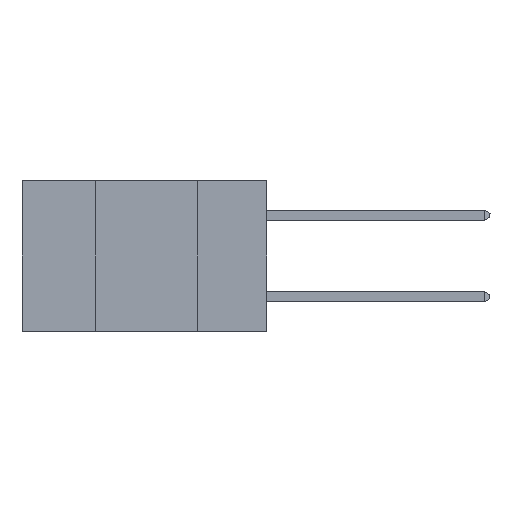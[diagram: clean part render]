
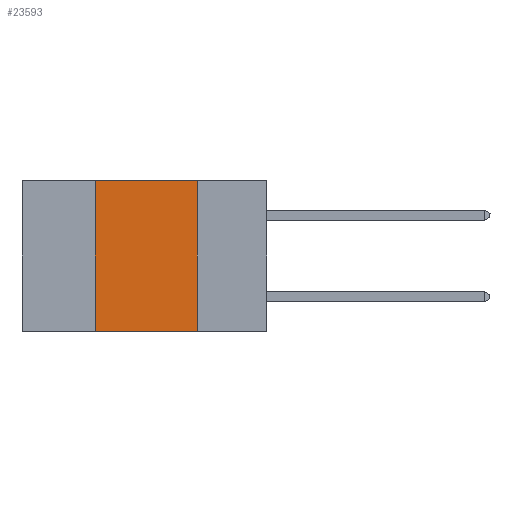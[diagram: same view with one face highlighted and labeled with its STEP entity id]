
A CAD part, left-side view. The second image highlights one B-rep face of the part: STEP entity #23593.
In plain terms, the highlighted planar face has unit normal (-1, 0, 0).
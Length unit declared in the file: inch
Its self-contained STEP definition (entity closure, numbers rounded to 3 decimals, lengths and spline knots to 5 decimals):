
#224 = EDGE_CURVE ( 'NONE', #19193, #25622, #569, .T. ) ;
#418 = ORIENTED_EDGE ( 'NONE', *, *, #20161, .F. ) ;
#569 = LINE ( 'NONE', #13970, #28613 ) ;
#1901 = CARTESIAN_POINT ( 'NONE',  ( 0., 0.42, -0.37 ) ) ;
#2568 = CARTESIAN_POINT ( 'NONE',  ( 0., 0.17, -0.37 ) ) ;
#2812 = EDGE_LOOP ( 'NONE', ( #418, #16305, #35563, #21832 ) ) ;
#4475 = CARTESIAN_POINT ( 'NONE',  ( 0., 0.6, 0. ) ) ;
#4681 = EDGE_CURVE ( 'NONE', #19193, #18682, #34011, .T. ) ;
#4736 = DIRECTION ( 'NONE',  ( 0., 0., -1. ) ) ;
#6014 = DIRECTION ( 'NONE',  ( 0., 0., -1. ) ) ;
#7960 = CARTESIAN_POINT ( 'NONE',  ( 0., 0.42, 0. ) ) ;
#8707 = CARTESIAN_POINT ( 'NONE',  ( 0., 0.17, 0. ) ) ;
#9124 = CARTESIAN_POINT ( 'NONE',  ( 0., 0.6, -0.37 ) ) ;
#9459 = CARTESIAN_POINT ( 'NONE',  ( 0., 0.17, 0. ) ) ;
#9792 = EDGE_CURVE ( 'NONE', #25622, #32981, #25194, .T. ) ;
#10490 = DIRECTION ( 'NONE',  ( 0., -1., 0. ) ) ;
#13970 = CARTESIAN_POINT ( 'NONE',  ( 0., 0.42, 0. ) ) ;
#14282 = DIRECTION ( 'NONE',  ( 1., 0., 0. ) ) ;
#16305 = ORIENTED_EDGE ( 'NONE', *, *, #9792, .F. ) ;
#16681 = VECTOR ( 'NONE', #10490, 39.37008 ) ;
#17497 = VECTOR ( 'NONE', #37949, 39.37008 ) ;
#18682 = VERTEX_POINT ( 'NONE', #2568 ) ;
#19193 = VERTEX_POINT ( 'NONE', #1901 ) ;
#20161 = EDGE_CURVE ( 'NONE', #32981, #18682, #33268, .T. ) ;
#21832 = ORIENTED_EDGE ( 'NONE', *, *, #4681, .T. ) ;
#23593 = ADVANCED_FACE ( 'NONE', ( #38097 ), #37079, .F. ) ;
#25142 = AXIS2_PLACEMENT_3D ( 'NONE', #30291, #14282, #4736 ) ;
#25194 = LINE ( 'NONE', #4475, #16681 ) ;
#25622 = VERTEX_POINT ( 'NONE', #7960 ) ;
#28613 = VECTOR ( 'NONE', #35464, 39.37008 ) ;
#30291 = CARTESIAN_POINT ( 'NONE',  ( 0., 0.6, 0. ) ) ;
#32981 = VERTEX_POINT ( 'NONE', #9459 ) ;
#33268 = LINE ( 'NONE', #8707, #38378 ) ;
#34011 = LINE ( 'NONE', #9124, #17497 ) ;
#35464 = DIRECTION ( 'NONE',  ( 0., 0., 1. ) ) ;
#35563 = ORIENTED_EDGE ( 'NONE', *, *, #224, .F. ) ;
#37079 = PLANE ( 'NONE',  #25142 ) ;
#37949 = DIRECTION ( 'NONE',  ( 0., -1., 0. ) ) ;
#38097 = FACE_OUTER_BOUND ( 'NONE', #2812, .T. ) ;
#38378 = VECTOR ( 'NONE', #6014, 39.37008 ) ;
